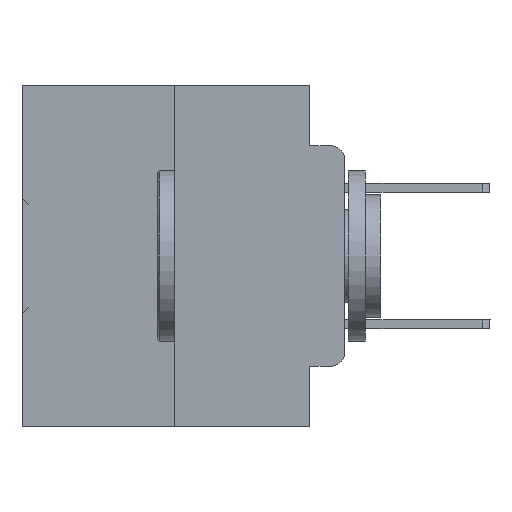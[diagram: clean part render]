
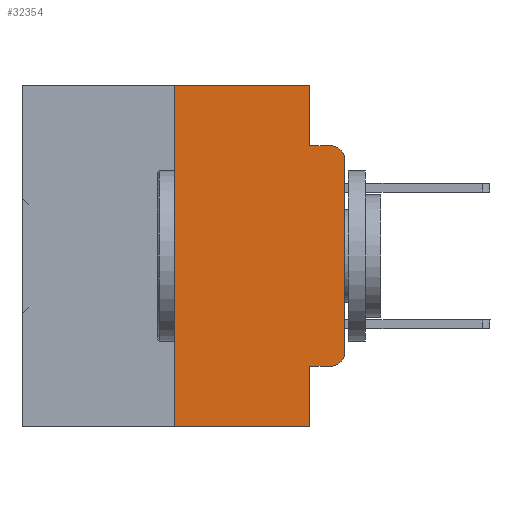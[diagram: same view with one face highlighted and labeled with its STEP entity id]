
A CAD part, left-side view. The second image highlights one B-rep face of the part: STEP entity #32354.
In plain terms, the highlighted planar face has unit normal (-1, 0, 0).
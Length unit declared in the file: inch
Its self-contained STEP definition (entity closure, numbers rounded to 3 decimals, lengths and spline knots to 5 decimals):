
#99 = EDGE_CURVE ( 'NONE', #11340, #2399, #20840, .T. ) ;
#412 = DIRECTION ( 'NONE',  ( 0., -1., 0. ) ) ;
#626 = CARTESIAN_POINT ( 'NONE',  ( 0., 0., 0. ) ) ;
#1289 = VERTEX_POINT ( 'NONE', #8627 ) ;
#2399 = VERTEX_POINT ( 'NONE', #12200 ) ;
#2816 = DIRECTION ( 'NONE',  ( 0., -1., 0. ) ) ;
#3103 = DIRECTION ( 'NONE',  ( 0., 0., -1. ) ) ;
#4112 = VECTOR ( 'NONE', #13086, 39.37008 ) ;
#4240 = VECTOR ( 'NONE', #12659, 39.37008 ) ;
#4358 = CARTESIAN_POINT ( 'NONE',  ( 0., 0.051, 0. ) ) ;
#4937 = VECTOR ( 'NONE', #3103, 39.37008 ) ;
#5602 = CIRCLE ( 'NONE', #20501, 0.02 ) ;
#5779 = DIRECTION ( 'NONE',  ( -1., 0., 0. ) ) ;
#6264 = CARTESIAN_POINT ( 'NONE',  ( 0., 0.25, -0.5 ) ) ;
#6382 = CARTESIAN_POINT ( 'NONE',  ( 0., 0.051, 0. ) ) ;
#6607 = CARTESIAN_POINT ( 'NONE',  ( 0., 0.473, -0.5 ) ) ;
#6953 = CARTESIAN_POINT ( 'NONE',  ( 0., 0.02, -0.1085 ) ) ;
#7131 = DIRECTION ( 'NONE',  ( 0., -1., 0. ) ) ;
#7515 = LINE ( 'NONE', #30878, #30066 ) ;
#8097 = VERTEX_POINT ( 'NONE', #13427 ) ;
#8120 = ORIENTED_EDGE ( 'NONE', *, *, #34973, .F. ) ;
#8284 = ORIENTED_EDGE ( 'NONE', *, *, #17765, .T. ) ;
#8342 = EDGE_CURVE ( 'NONE', #1289, #2399, #5602, .T. ) ;
#8367 = CARTESIAN_POINT ( 'NONE',  ( 0., 0., -0.3915 ) ) ;
#8627 = CARTESIAN_POINT ( 'NONE',  ( 0., 0., -0.1085 ) ) ;
#8874 = DIRECTION ( 'NONE',  ( 1., 0., 0. ) ) ;
#9139 = ORIENTED_EDGE ( 'NONE', *, *, #20213, .T. ) ;
#9379 = CARTESIAN_POINT ( 'NONE',  ( 0., 0.051, -0.5 ) ) ;
#10168 = ORIENTED_EDGE ( 'NONE', *, *, #15836, .F. ) ;
#10906 = VERTEX_POINT ( 'NONE', #8367 ) ;
#11340 = VERTEX_POINT ( 'NONE', #35539 ) ;
#11821 = DIRECTION ( 'NONE',  ( 0., 0., -1. ) ) ;
#11967 = EDGE_CURVE ( 'NONE', #22073, #8097, #7515, .T. ) ;
#12186 = AXIS2_PLACEMENT_3D ( 'NONE', #30272, #8874, #29691 ) ;
#12200 = CARTESIAN_POINT ( 'NONE',  ( 0., 0.02, -0.0885 ) ) ;
#12276 = LINE ( 'NONE', #626, #4240 ) ;
#12659 = DIRECTION ( 'NONE',  ( 0., 0., 1. ) ) ;
#12945 = VECTOR ( 'NONE', #19358, 39.37008 ) ;
#12961 = ORIENTED_EDGE ( 'NONE', *, *, #11967, .F. ) ;
#13086 = DIRECTION ( 'NONE',  ( 0., 0., -1. ) ) ;
#13427 = CARTESIAN_POINT ( 'NONE',  ( 0., 0.051, 0. ) ) ;
#14476 = ORIENTED_EDGE ( 'NONE', *, *, #8342, .T. ) ;
#14775 = DIRECTION ( 'NONE',  ( 0., -1., 0. ) ) ;
#15504 = DIRECTION ( 'NONE',  ( 0., 0., -1. ) ) ;
#15836 = EDGE_CURVE ( 'NONE', #8097, #11340, #18917, .T. ) ;
#15907 = DIRECTION ( 'NONE',  ( -1., 0., 0. ) ) ;
#16737 = AXIS2_PLACEMENT_3D ( 'NONE', #31514, #5779, #11821 ) ;
#17011 = ORIENTED_EDGE ( 'NONE', *, *, #36555, .F. ) ;
#17040 = ORIENTED_EDGE ( 'NONE', *, *, #17343, .T. ) ;
#17124 = CARTESIAN_POINT ( 'NONE',  ( 0., 0.051, -0.4115 ) ) ;
#17343 = EDGE_CURVE ( 'NONE', #10906, #1289, #12276, .T. ) ;
#17765 = EDGE_CURVE ( 'NONE', #23263, #26441, #29583, .T. ) ;
#18917 = LINE ( 'NONE', #4358, #4112 ) ;
#19358 = DIRECTION ( 'NONE',  ( 0., 0., 1. ) ) ;
#20213 = EDGE_CURVE ( 'NONE', #26441, #10906, #29802, .T. ) ;
#20501 = AXIS2_PLACEMENT_3D ( 'NONE', #6953, #15907, #15504 ) ;
#20840 = LINE ( 'NONE', #27038, #24397 ) ;
#21298 = VERTEX_POINT ( 'NONE', #9379 ) ;
#22073 = VERTEX_POINT ( 'NONE', #30445 ) ;
#23263 = VERTEX_POINT ( 'NONE', #32663 ) ;
#24397 = VECTOR ( 'NONE', #2816, 39.37008 ) ;
#26441 = VERTEX_POINT ( 'NONE', #29863 ) ;
#27038 = CARTESIAN_POINT ( 'NONE',  ( 0., 0.051, -0.0885 ) ) ;
#27196 = LINE ( 'NONE', #6607, #29597 ) ;
#29545 = ORIENTED_EDGE ( 'NONE', *, *, #99, .F. ) ;
#29583 = LINE ( 'NONE', #17124, #32626 ) ;
#29597 = VECTOR ( 'NONE', #412, 39.37008 ) ;
#29691 = DIRECTION ( 'NONE',  ( 0., 0., -1. ) ) ;
#29802 = CIRCLE ( 'NONE', #16737, 0.02 ) ;
#29863 = CARTESIAN_POINT ( 'NONE',  ( 0., 0.02, -0.4115 ) ) ;
#30066 = VECTOR ( 'NONE', #7131, 39.37008 ) ;
#30181 = EDGE_CURVE ( 'NONE', #38355, #21298, #27196, .T. ) ;
#30272 = CARTESIAN_POINT ( 'NONE',  ( 0., 0.473, 0. ) ) ;
#30445 = CARTESIAN_POINT ( 'NONE',  ( 0., 0.25, 0. ) ) ;
#30878 = CARTESIAN_POINT ( 'NONE',  ( 0., 0.473, 0. ) ) ;
#31259 = LINE ( 'NONE', #36505, #12945 ) ;
#31514 = CARTESIAN_POINT ( 'NONE',  ( 0., 0.02, -0.3915 ) ) ;
#32354 = ADVANCED_FACE ( 'NONE', ( #33183 ), #35906, .F. ) ;
#32626 = VECTOR ( 'NONE', #14775, 39.37008 ) ;
#32663 = CARTESIAN_POINT ( 'NONE',  ( 0., 0.051, -0.4115 ) ) ;
#32685 = LINE ( 'NONE', #6382, #4937 ) ;
#33183 = FACE_OUTER_BOUND ( 'NONE', #34308, .T. ) ;
#33716 = ORIENTED_EDGE ( 'NONE', *, *, #30181, .T. ) ;
#34308 = EDGE_LOOP ( 'NONE', ( #17040, #14476, #29545, #10168, #12961, #17011, #33716, #8120, #8284, #9139 ) ) ;
#34973 = EDGE_CURVE ( 'NONE', #23263, #21298, #32685, .T. ) ;
#35539 = CARTESIAN_POINT ( 'NONE',  ( 0., 0.051, -0.0885 ) ) ;
#35906 = PLANE ( 'NONE',  #12186 ) ;
#36505 = CARTESIAN_POINT ( 'NONE',  ( 0., 0.25, 0. ) ) ;
#36555 = EDGE_CURVE ( 'NONE', #38355, #22073, #31259, .T. ) ;
#38355 = VERTEX_POINT ( 'NONE', #6264 ) ;
